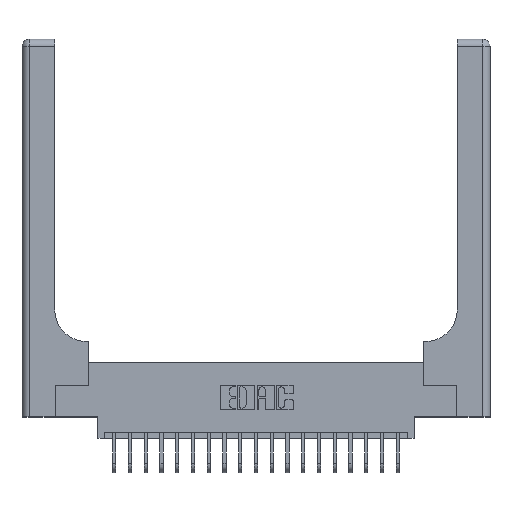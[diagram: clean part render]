
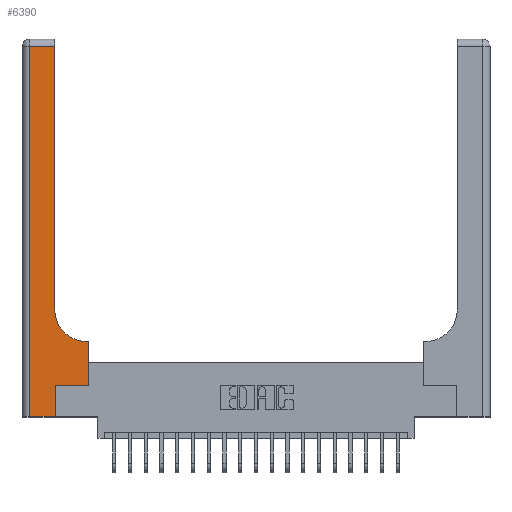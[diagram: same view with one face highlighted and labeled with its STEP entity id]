
A CAD part, top view. The second image highlights one B-rep face of the part: STEP entity #6390.
In plain terms, the highlighted planar face has unit normal (0, 0, 1).
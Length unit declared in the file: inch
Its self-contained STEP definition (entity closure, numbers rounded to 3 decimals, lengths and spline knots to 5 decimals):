
#251 = VECTOR ( 'NONE', #3490, 39.37008 ) ;
#625 = LINE ( 'NONE', #15455, #14296 ) ;
#1272 = CARTESIAN_POINT ( 'NONE',  ( 0.51, 0.85, 0.37 ) ) ;
#1826 = CARTESIAN_POINT ( 'NONE',  ( 0.528, 0.25, 0.37 ) ) ;
#2313 = EDGE_CURVE ( 'NONE', #7923, #20602, #7893, .T. ) ;
#2346 = VERTEX_POINT ( 'NONE', #16351 ) ;
#2511 = CARTESIAN_POINT ( 'NONE',  ( 0.265, 0.25, 0.37 ) ) ;
#2786 = CARTESIAN_POINT ( 'NONE',  ( 0.51, 0.6, 0.37 ) ) ;
#2792 = ORIENTED_EDGE ( 'NONE', *, *, #8879, .T. ) ;
#3309 = VERTEX_POINT ( 'NONE', #8758 ) ;
#3376 = ORIENTED_EDGE ( 'NONE', *, *, #11770, .T. ) ;
#3451 = EDGE_LOOP ( 'NONE', ( #2792, #11806, #6053, #8180, #5691, #3376, #6398, #9979, #6809 ) ) ;
#3490 = DIRECTION ( 'NONE',  ( 0., 1., 0. ) ) ;
#3642 = LINE ( 'NONE', #20132, #21681 ) ;
#3792 = DIRECTION ( 'NONE',  ( -1., 0., 0. ) ) ;
#3969 = EDGE_CURVE ( 'NONE', #3309, #2346, #14412, .T. ) ;
#4037 = AXIS2_PLACEMENT_3D ( 'NONE', #1272, #13196, #9750 ) ;
#4418 = CARTESIAN_POINT ( 'NONE',  ( 0.26, 0.85, 0.37 ) ) ;
#4738 = DIRECTION ( 'NONE',  ( 0., 1., 0. ) ) ;
#4840 = EDGE_CURVE ( 'NONE', #20602, #10140, #5593, .T. ) ;
#5334 = LINE ( 'NONE', #7730, #13744 ) ;
#5593 = LINE ( 'NONE', #19472, #21988 ) ;
#5691 = ORIENTED_EDGE ( 'NONE', *, *, #18232, .T. ) ;
#6053 = ORIENTED_EDGE ( 'NONE', *, *, #10384, .T. ) ;
#6390 = ADVANCED_FACE ( 'NONE', ( #7985 ), #12875, .F. ) ;
#6398 = ORIENTED_EDGE ( 'NONE', *, *, #2313, .T. ) ;
#6809 = ORIENTED_EDGE ( 'NONE', *, *, #11939, .T. ) ;
#7500 = CARTESIAN_POINT ( 'NONE',  ( 0., 0., 0.37 ) ) ;
#7675 = DIRECTION ( 'NONE',  ( -1., 0., 0. ) ) ;
#7730 = CARTESIAN_POINT ( 'NONE',  ( 0.26, 3., 0.37 ) ) ;
#7775 = DIRECTION ( 'NONE',  ( 1., 0., 0. ) ) ;
#7893 = LINE ( 'NONE', #15482, #251 ) ;
#7923 = VERTEX_POINT ( 'NONE', #1826 ) ;
#7985 = FACE_OUTER_BOUND ( 'NONE', #3451, .T. ) ;
#8000 = LINE ( 'NONE', #18652, #17595 ) ;
#8180 = ORIENTED_EDGE ( 'NONE', *, *, #3969, .T. ) ;
#8541 = CARTESIAN_POINT ( 'NONE',  ( 0.265, 0.25, 0.37 ) ) ;
#8745 = CIRCLE ( 'NONE', #4037, 0.25 ) ;
#8758 = CARTESIAN_POINT ( 'NONE',  ( 0.06, 0., 0.37 ) ) ;
#8879 = EDGE_CURVE ( 'NONE', #13197, #12082, #5334, .T. ) ;
#9121 = DIRECTION ( 'NONE',  ( 1., 0., 0. ) ) ;
#9750 = DIRECTION ( 'NONE',  ( 1., 0., 0. ) ) ;
#9913 = CARTESIAN_POINT ( 'NONE',  ( 0.06, 2.94, 0.37 ) ) ;
#9979 = ORIENTED_EDGE ( 'NONE', *, *, #4840, .T. ) ;
#10140 = VERTEX_POINT ( 'NONE', #2786 ) ;
#10147 = EDGE_CURVE ( 'NONE', #12082, #20554, #3642, .T. ) ;
#10384 = EDGE_CURVE ( 'NONE', #20554, #3309, #625, .T. ) ;
#11704 = DIRECTION ( 'NONE',  ( -1., 0., 0. ) ) ;
#11738 = AXIS2_PLACEMENT_3D ( 'NONE', #16377, #14643, #7675 ) ;
#11770 = EDGE_CURVE ( 'NONE', #18880, #7923, #17757, .T. ) ;
#11806 = ORIENTED_EDGE ( 'NONE', *, *, #10147, .T. ) ;
#11939 = EDGE_CURVE ( 'NONE', #10140, #13197, #8745, .T. ) ;
#11994 = VECTOR ( 'NONE', #7775, 39.37008 ) ;
#12082 = VERTEX_POINT ( 'NONE', #20833 ) ;
#12875 = PLANE ( 'NONE',  #11738 ) ;
#13196 = DIRECTION ( 'NONE',  ( 0., 0., -1. ) ) ;
#13197 = VERTEX_POINT ( 'NONE', #4418 ) ;
#13744 = VECTOR ( 'NONE', #16506, 39.37008 ) ;
#13859 = VECTOR ( 'NONE', #9121, 39.37008 ) ;
#14296 = VECTOR ( 'NONE', #17276, 39.37008 ) ;
#14412 = LINE ( 'NONE', #7500, #13859 ) ;
#14643 = DIRECTION ( 'NONE',  ( 0., 0., -1. ) ) ;
#15455 = CARTESIAN_POINT ( 'NONE',  ( 0.06, 3., 0.37 ) ) ;
#15482 = CARTESIAN_POINT ( 'NONE',  ( 0.528, 0.25, 0.37 ) ) ;
#15572 = CARTESIAN_POINT ( 'NONE',  ( 0.528, 0.6, 0.37 ) ) ;
#16351 = CARTESIAN_POINT ( 'NONE',  ( 0.265, 0., 0.37 ) ) ;
#16377 = CARTESIAN_POINT ( 'NONE',  ( 0., 3., 0.37 ) ) ;
#16506 = DIRECTION ( 'NONE',  ( 0., 1., 0. ) ) ;
#17276 = DIRECTION ( 'NONE',  ( 0., -1., 0. ) ) ;
#17595 = VECTOR ( 'NONE', #4738, 39.37008 ) ;
#17757 = LINE ( 'NONE', #2511, #11994 ) ;
#18232 = EDGE_CURVE ( 'NONE', #2346, #18880, #8000, .T. ) ;
#18652 = CARTESIAN_POINT ( 'NONE',  ( 0.265, 0., 0.37 ) ) ;
#18880 = VERTEX_POINT ( 'NONE', #8541 ) ;
#19472 = CARTESIAN_POINT ( 'NONE',  ( 0.26, 0.6, 0.37 ) ) ;
#20132 = CARTESIAN_POINT ( 'NONE',  ( 0., 2.94, 0.37 ) ) ;
#20554 = VERTEX_POINT ( 'NONE', #9913 ) ;
#20602 = VERTEX_POINT ( 'NONE', #15572 ) ;
#20833 = CARTESIAN_POINT ( 'NONE',  ( 0.26, 2.94, 0.37 ) ) ;
#21681 = VECTOR ( 'NONE', #11704, 39.37008 ) ;
#21988 = VECTOR ( 'NONE', #3792, 39.37008 ) ;
